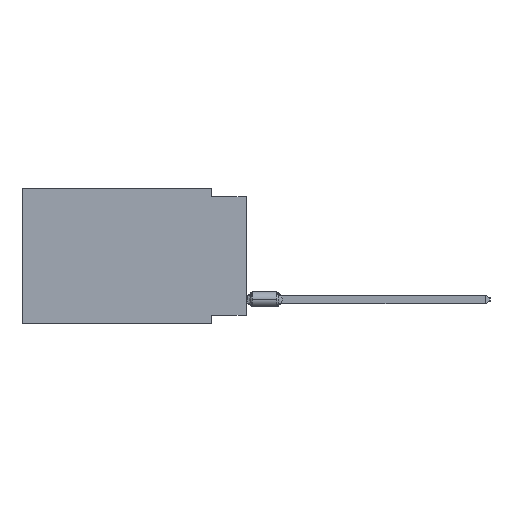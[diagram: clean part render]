
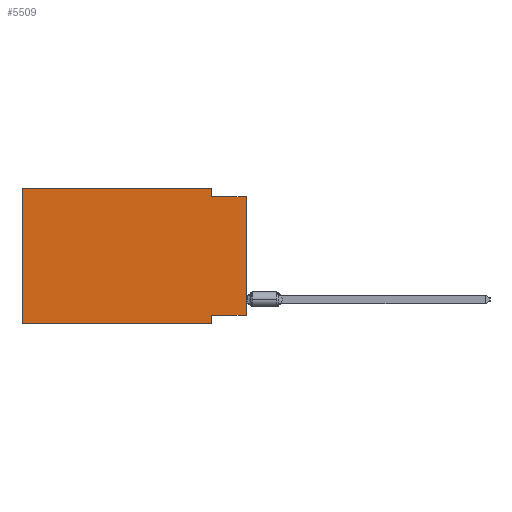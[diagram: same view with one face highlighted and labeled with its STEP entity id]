
A CAD part, left-side view. The second image highlights one B-rep face of the part: STEP entity #5509.
In plain terms, the highlighted planar face has unit normal (-1, 0, 0).
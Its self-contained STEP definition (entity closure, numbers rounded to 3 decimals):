
#886 = ORIENTED_EDGE ( 'NONE', *, *, #30963, .T. ) ;
#1990 = LINE ( 'NONE', #5591, #43278 ) ;
#2145 = ORIENTED_EDGE ( 'NONE', *, *, #4291, .F. ) ;
#2206 = CARTESIAN_POINT ( 'NONE',  ( 0., 16.383, 0. ) ) ;
#3201 = VECTOR ( 'NONE', #39393, 1000. ) ;
#3770 = VERTEX_POINT ( 'NONE', #10805 ) ;
#4015 = CARTESIAN_POINT ( 'NONE',  ( 0., 2.54, -9.906 ) ) ;
#4133 = EDGE_CURVE ( 'NONE', #31329, #15396, #17257, .T. ) ;
#4291 = EDGE_CURVE ( 'NONE', #3770, #12794, #8271, .T. ) ;
#4772 = LINE ( 'NONE', #35687, #4834 ) ;
#4834 = VECTOR ( 'NONE', #36138, 1000. ) ;
#5509 = ADVANCED_FACE ( 'NONE', ( #19461 ), #32695, .F. ) ;
#5591 = CARTESIAN_POINT ( 'NONE',  ( 0., 0., -0.635 ) ) ;
#6972 = CARTESIAN_POINT ( 'NONE',  ( 0., 16.383, 0. ) ) ;
#8271 = LINE ( 'NONE', #42099, #3201 ) ;
#9298 = EDGE_CURVE ( 'NONE', #15396, #20522, #20577, .T. ) ;
#10805 = CARTESIAN_POINT ( 'NONE',  ( 0., 0., -9.271 ) ) ;
#12098 = ORIENTED_EDGE ( 'NONE', *, *, #34913, .F. ) ;
#12794 = VERTEX_POINT ( 'NONE', #39925 ) ;
#12842 = LINE ( 'NONE', #30548, #38368 ) ;
#13182 = DIRECTION ( 'NONE',  ( 0., 0., -1. ) ) ;
#14183 = CARTESIAN_POINT ( 'NONE',  ( 0., 16.383, -9.906 ) ) ;
#14215 = CARTESIAN_POINT ( 'NONE',  ( 0., 2.54, -0.635 ) ) ;
#15396 = VERTEX_POINT ( 'NONE', #30524 ) ;
#16371 = LINE ( 'NONE', #21014, #26527 ) ;
#16542 = ORIENTED_EDGE ( 'NONE', *, *, #23119, .T. ) ;
#17257 = LINE ( 'NONE', #6972, #22528 ) ;
#17526 = ORIENTED_EDGE ( 'NONE', *, *, #29654, .F. ) ;
#19461 = FACE_OUTER_BOUND ( 'NONE', #20587, .T. ) ;
#20444 = AXIS2_PLACEMENT_3D ( 'NONE', #2206, #26425, #13182 ) ;
#20522 = VERTEX_POINT ( 'NONE', #39624 ) ;
#20577 = LINE ( 'NONE', #34033, #25675 ) ;
#20587 = EDGE_LOOP ( 'NONE', ( #886, #12098, #17526, #40895, #40681, #16542, #23023, #2145 ) ) ;
#20672 = DIRECTION ( 'NONE',  ( 0., 0., -1. ) ) ;
#21014 = CARTESIAN_POINT ( 'NONE',  ( 0., 2.54, 0. ) ) ;
#21062 = DIRECTION ( 'NONE',  ( 0., 0., 1. ) ) ;
#22528 = VECTOR ( 'NONE', #21062, 1000. ) ;
#23023 = ORIENTED_EDGE ( 'NONE', *, *, #37895, .F. ) ;
#23119 = EDGE_CURVE ( 'NONE', #31329, #31236, #23599, .T. ) ;
#23599 = LINE ( 'NONE', #14183, #25476 ) ;
#24850 = VERTEX_POINT ( 'NONE', #26356 ) ;
#25476 = VECTOR ( 'NONE', #37278, 1000. ) ;
#25675 = VECTOR ( 'NONE', #31341, 1000. ) ;
#26356 = CARTESIAN_POINT ( 'NONE',  ( 0., 0., -0.635 ) ) ;
#26425 = DIRECTION ( 'NONE',  ( 1., 0., 0. ) ) ;
#26527 = VECTOR ( 'NONE', #30491, 1000. ) ;
#29116 = DIRECTION ( 'NONE',  ( 0., -1., 0. ) ) ;
#29654 = EDGE_CURVE ( 'NONE', #20522, #36442, #16371, .T. ) ;
#30491 = DIRECTION ( 'NONE',  ( 0., 0., -1. ) ) ;
#30524 = CARTESIAN_POINT ( 'NONE',  ( 0., 16.383, 0. ) ) ;
#30548 = CARTESIAN_POINT ( 'NONE',  ( 0., 2.54, -9.906 ) ) ;
#30963 = EDGE_CURVE ( 'NONE', #3770, #24850, #4772, .T. ) ;
#31236 = VERTEX_POINT ( 'NONE', #4015 ) ;
#31329 = VERTEX_POINT ( 'NONE', #39594 ) ;
#31341 = DIRECTION ( 'NONE',  ( 0., -1., 0. ) ) ;
#32695 = PLANE ( 'NONE',  #20444 ) ;
#34033 = CARTESIAN_POINT ( 'NONE',  ( 0., 16.383, 0. ) ) ;
#34913 = EDGE_CURVE ( 'NONE', #36442, #24850, #1990, .T. ) ;
#35687 = CARTESIAN_POINT ( 'NONE',  ( 0., 0., 0. ) ) ;
#36138 = DIRECTION ( 'NONE',  ( 0., 0., 1. ) ) ;
#36442 = VERTEX_POINT ( 'NONE', #14215 ) ;
#37278 = DIRECTION ( 'NONE',  ( 0., -1., 0. ) ) ;
#37895 = EDGE_CURVE ( 'NONE', #12794, #31236, #12842, .T. ) ;
#38368 = VECTOR ( 'NONE', #20672, 1000. ) ;
#39393 = DIRECTION ( 'NONE',  ( 0., 1., 0. ) ) ;
#39594 = CARTESIAN_POINT ( 'NONE',  ( 0., 16.383, -9.906 ) ) ;
#39624 = CARTESIAN_POINT ( 'NONE',  ( 0., 2.54, 0. ) ) ;
#39925 = CARTESIAN_POINT ( 'NONE',  ( 0., 2.54, -9.271 ) ) ;
#40681 = ORIENTED_EDGE ( 'NONE', *, *, #4133, .F. ) ;
#40895 = ORIENTED_EDGE ( 'NONE', *, *, #9298, .F. ) ;
#42099 = CARTESIAN_POINT ( 'NONE',  ( 0., 0., -9.271 ) ) ;
#43278 = VECTOR ( 'NONE', #29116, 1000. ) ;
